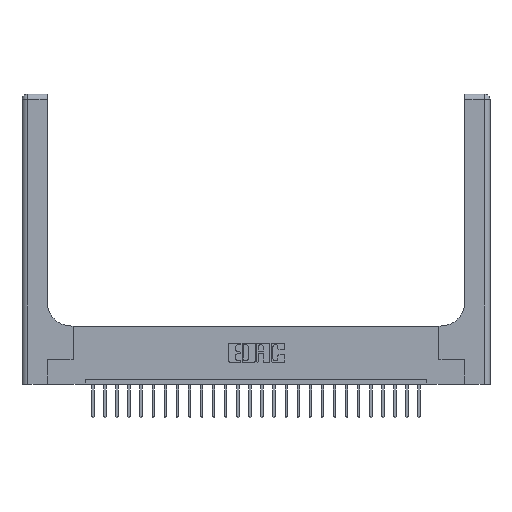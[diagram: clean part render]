
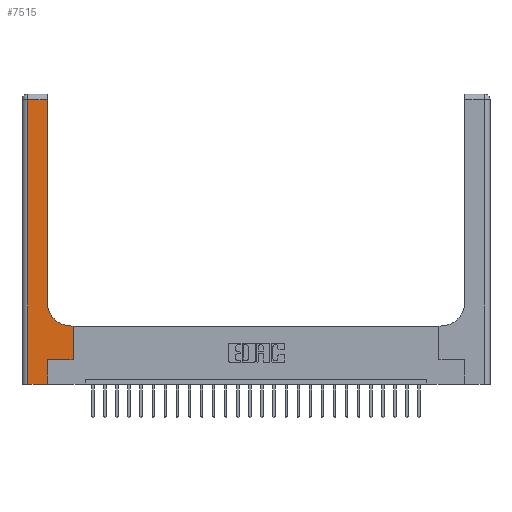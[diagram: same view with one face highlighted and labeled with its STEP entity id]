
A CAD part, top view. The second image highlights one B-rep face of the part: STEP entity #7515.
In plain terms, the highlighted planar face has unit normal (0, 0, 1).
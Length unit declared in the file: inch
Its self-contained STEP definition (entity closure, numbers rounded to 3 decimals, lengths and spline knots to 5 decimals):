
#61 = CARTESIAN_POINT ( 'NONE',  ( 0.26, 2.94, 0.37 ) ) ;
#608 = CARTESIAN_POINT ( 'NONE',  ( 0., 3., 0.37 ) ) ;
#904 = CARTESIAN_POINT ( 'NONE',  ( 0.265, 0., 0.37 ) ) ;
#1153 = ORIENTED_EDGE ( 'NONE', *, *, #11108, .T. ) ;
#2441 = CARTESIAN_POINT ( 'NONE',  ( 0.528, 0.25, 0.37 ) ) ;
#2721 = CARTESIAN_POINT ( 'NONE',  ( 0.26, 0.6, 0.37 ) ) ;
#3128 = VERTEX_POINT ( 'NONE', #23495 ) ;
#3198 = CARTESIAN_POINT ( 'NONE',  ( 0.265, 0.25, 0.37 ) ) ;
#3304 = LINE ( 'NONE', #5581, #10742 ) ;
#3478 = ORIENTED_EDGE ( 'NONE', *, *, #12365, .T. ) ;
#4440 = DIRECTION ( 'NONE',  ( -1., 0., 0. ) ) ;
#4620 = VERTEX_POINT ( 'NONE', #18194 ) ;
#4626 = AXIS2_PLACEMENT_3D ( 'NONE', #608, #15738, #4440 ) ;
#5581 = CARTESIAN_POINT ( 'NONE',  ( 0., 2.94, 0.37 ) ) ;
#5932 = VERTEX_POINT ( 'NONE', #16042 ) ;
#5968 = AXIS2_PLACEMENT_3D ( 'NONE', #20012, #23804, #12486 ) ;
#6890 = CARTESIAN_POINT ( 'NONE',  ( 0.26, 3., 0.37 ) ) ;
#7251 = DIRECTION ( 'NONE',  ( 0., 1., 0. ) ) ;
#7515 = ADVANCED_FACE ( 'NONE', ( #9516 ), #11929, .F. ) ;
#8733 = EDGE_CURVE ( 'NONE', #15989, #5932, #19755, .T. ) ;
#9132 = ORIENTED_EDGE ( 'NONE', *, *, #18144, .T. ) ;
#9407 = EDGE_CURVE ( 'NONE', #5932, #4620, #16466, .T. ) ;
#9516 = FACE_OUTER_BOUND ( 'NONE', #9735, .T. ) ;
#9735 = EDGE_LOOP ( 'NONE', ( #9132, #3478, #13468, #15858, #16052, #1153, #14520, #16896, #17707 ) ) ;
#10538 = CARTESIAN_POINT ( 'NONE',  ( 0.06, 0., 0.37 ) ) ;
#10622 = LINE ( 'NONE', #2441, #14460 ) ;
#10742 = VECTOR ( 'NONE', #12904, 39.37008 ) ;
#11108 = EDGE_CURVE ( 'NONE', #4620, #16197, #23163, .T. ) ;
#11578 = DIRECTION ( 'NONE',  ( 1., 0., 0. ) ) ;
#11655 = CIRCLE ( 'NONE', #5968, 0.25 ) ;
#11929 = PLANE ( 'NONE',  #4626 ) ;
#12365 = EDGE_CURVE ( 'NONE', #16452, #3128, #3304, .T. ) ;
#12482 = EDGE_CURVE ( 'NONE', #3128, #15989, #23391, .T. ) ;
#12486 = DIRECTION ( 'NONE',  ( 1., 0., 0. ) ) ;
#12904 = DIRECTION ( 'NONE',  ( -1., 0., 0. ) ) ;
#13090 = VERTEX_POINT ( 'NONE', #16662 ) ;
#13326 = CARTESIAN_POINT ( 'NONE',  ( 0.528, 0.25, 0.37 ) ) ;
#13468 = ORIENTED_EDGE ( 'NONE', *, *, #12482, .T. ) ;
#14063 = EDGE_CURVE ( 'NONE', #22667, #15110, #11655, .T. ) ;
#14119 = VECTOR ( 'NONE', #11578, 39.37008 ) ;
#14398 = CARTESIAN_POINT ( 'NONE',  ( 0., 0., 0.37 ) ) ;
#14460 = VECTOR ( 'NONE', #19302, 39.37008 ) ;
#14520 = ORIENTED_EDGE ( 'NONE', *, *, #21962, .T. ) ;
#14837 = DIRECTION ( 'NONE',  ( 1., 0., 0. ) ) ;
#14971 = CARTESIAN_POINT ( 'NONE',  ( 0.06, 3., 0.37 ) ) ;
#15110 = VERTEX_POINT ( 'NONE', #23075 ) ;
#15363 = VECTOR ( 'NONE', #23907, 39.37008 ) ;
#15738 = DIRECTION ( 'NONE',  ( 0., 0., -1. ) ) ;
#15858 = ORIENTED_EDGE ( 'NONE', *, *, #8733, .T. ) ;
#15989 = VERTEX_POINT ( 'NONE', #10538 ) ;
#16042 = CARTESIAN_POINT ( 'NONE',  ( 0.265, 0., 0.37 ) ) ;
#16052 = ORIENTED_EDGE ( 'NONE', *, *, #9407, .T. ) ;
#16197 = VERTEX_POINT ( 'NONE', #13326 ) ;
#16452 = VERTEX_POINT ( 'NONE', #61 ) ;
#16466 = LINE ( 'NONE', #904, #20633 ) ;
#16662 = CARTESIAN_POINT ( 'NONE',  ( 0.528, 0.6, 0.37 ) ) ;
#16896 = ORIENTED_EDGE ( 'NONE', *, *, #24217, .T. ) ;
#17623 = LINE ( 'NONE', #2721, #18481 ) ;
#17707 = ORIENTED_EDGE ( 'NONE', *, *, #14063, .T. ) ;
#18144 = EDGE_CURVE ( 'NONE', #15110, #16452, #20071, .T. ) ;
#18194 = CARTESIAN_POINT ( 'NONE',  ( 0.265, 0.25, 0.37 ) ) ;
#18438 = DIRECTION ( 'NONE',  ( 0., -1., 0. ) ) ;
#18481 = VECTOR ( 'NONE', #19728, 39.37008 ) ;
#18701 = CARTESIAN_POINT ( 'NONE',  ( 0.51, 0.6, 0.37 ) ) ;
#19302 = DIRECTION ( 'NONE',  ( 0., 1., 0. ) ) ;
#19728 = DIRECTION ( 'NONE',  ( -1., 0., 0. ) ) ;
#19755 = LINE ( 'NONE', #14398, #14119 ) ;
#20012 = CARTESIAN_POINT ( 'NONE',  ( 0.51, 0.85, 0.37 ) ) ;
#20071 = LINE ( 'NONE', #6890, #15363 ) ;
#20192 = VECTOR ( 'NONE', #18438, 39.37008 ) ;
#20633 = VECTOR ( 'NONE', #7251, 39.37008 ) ;
#21962 = EDGE_CURVE ( 'NONE', #16197, #13090, #10622, .T. ) ;
#22667 = VERTEX_POINT ( 'NONE', #18701 ) ;
#23075 = CARTESIAN_POINT ( 'NONE',  ( 0.26, 0.85, 0.37 ) ) ;
#23163 = LINE ( 'NONE', #3198, #23756 ) ;
#23391 = LINE ( 'NONE', #14971, #20192 ) ;
#23495 = CARTESIAN_POINT ( 'NONE',  ( 0.06, 2.94, 0.37 ) ) ;
#23756 = VECTOR ( 'NONE', #14837, 39.37008 ) ;
#23804 = DIRECTION ( 'NONE',  ( 0., 0., -1. ) ) ;
#23907 = DIRECTION ( 'NONE',  ( 0., 1., 0. ) ) ;
#24217 = EDGE_CURVE ( 'NONE', #13090, #22667, #17623, .T. ) ;
